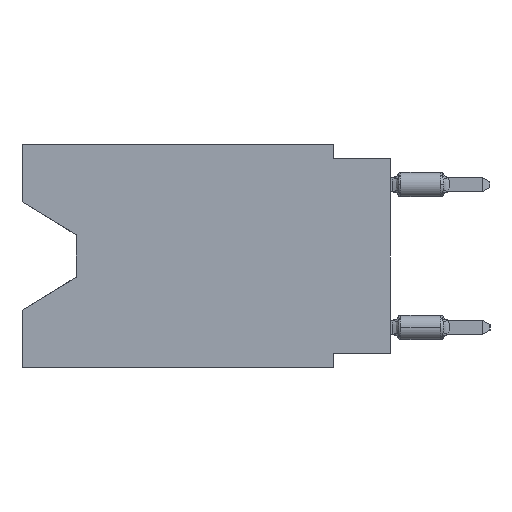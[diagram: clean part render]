
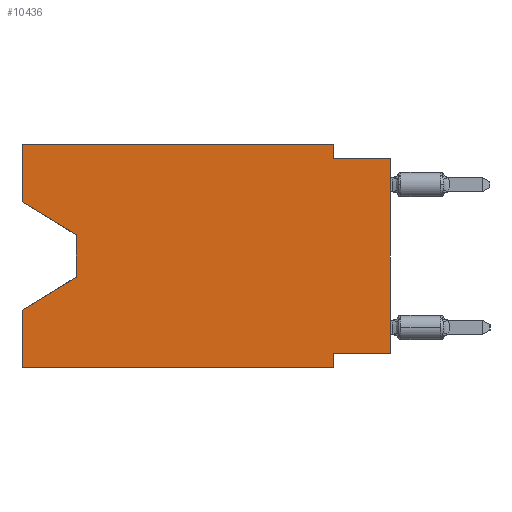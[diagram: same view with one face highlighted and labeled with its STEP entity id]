
A CAD part, left-side view. The second image highlights one B-rep face of the part: STEP entity #10436.
In plain terms, the highlighted planar face has unit normal (-1, 0, 0).
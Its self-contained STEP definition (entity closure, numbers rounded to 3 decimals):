
#299 = VECTOR ( 'NONE', #828, 1000. ) ;
#445 = EDGE_CURVE ( 'NONE', #14486, #13432, #19135, .T. ) ;
#828 = DIRECTION ( 'NONE',  ( 0., 0., -1. ) ) ;
#913 = DIRECTION ( 'NONE',  ( 1., 0., 0. ) ) ;
#1190 = EDGE_CURVE ( 'NONE', #18613, #14375, #9058, .T. ) ;
#1344 = ORIENTED_EDGE ( 'NONE', *, *, #16171, .T. ) ;
#1827 = CARTESIAN_POINT ( 'NONE',  ( 0., 0., 0. ) ) ;
#1930 = DIRECTION ( 'NONE',  ( 0., -1., 0. ) ) ;
#2116 = DIRECTION ( 'NONE',  ( 0., 1., 0. ) ) ;
#2745 = CARTESIAN_POINT ( 'NONE',  ( 0., 16.383, 0. ) ) ;
#3385 = CARTESIAN_POINT ( 'NONE',  ( 0., 2.54, -9.906 ) ) ;
#3682 = CARTESIAN_POINT ( 'NONE',  ( 0., 0., -0.635 ) ) ;
#4029 = PLANE ( 'NONE',  #21563 ) ;
#4590 = LINE ( 'NONE', #11635, #16053 ) ;
#4853 = EDGE_CURVE ( 'NONE', #9731, #14580, #8641, .T. ) ;
#5098 = ORIENTED_EDGE ( 'NONE', *, *, #14408, .F. ) ;
#5248 = CARTESIAN_POINT ( 'NONE',  ( 0., 13.97, -5.893 ) ) ;
#5390 = DIRECTION ( 'NONE',  ( 0., 0., 1. ) ) ;
#5468 = CARTESIAN_POINT ( 'NONE',  ( 0., 16.383, 0. ) ) ;
#5763 = FACE_OUTER_BOUND ( 'NONE', #14326, .T. ) ;
#5974 = DIRECTION ( 'NONE',  ( 0., -0.855, -0.519 ) ) ;
#6468 = VECTOR ( 'NONE', #14177, 1000. ) ;
#6736 = LINE ( 'NONE', #3385, #7605 ) ;
#6860 = VERTEX_POINT ( 'NONE', #8424 ) ;
#7077 = CARTESIAN_POINT ( 'NONE',  ( 0., 16.383, -2.546 ) ) ;
#7278 = ORIENTED_EDGE ( 'NONE', *, *, #10405, .F. ) ;
#7431 = DIRECTION ( 'NONE',  ( 0., 0.855, -0.519 ) ) ;
#7605 = VECTOR ( 'NONE', #15279, 1000. ) ;
#8278 = DIRECTION ( 'NONE',  ( 0., 0., -1. ) ) ;
#8424 = CARTESIAN_POINT ( 'NONE',  ( 0., 13.97, -4.013 ) ) ;
#8461 = ORIENTED_EDGE ( 'NONE', *, *, #18480, .T. ) ;
#8641 = LINE ( 'NONE', #10724, #6468 ) ;
#9058 = LINE ( 'NONE', #5248, #10427 ) ;
#9216 = DIRECTION ( 'NONE',  ( 0., -1., 0. ) ) ;
#9353 = ORIENTED_EDGE ( 'NONE', *, *, #19395, .F. ) ;
#9731 = VERTEX_POINT ( 'NONE', #22059 ) ;
#10322 = ORIENTED_EDGE ( 'NONE', *, *, #21096, .F. ) ;
#10364 = CARTESIAN_POINT ( 'NONE',  ( 0., 16.383, 0. ) ) ;
#10405 = EDGE_CURVE ( 'NONE', #14882, #22396, #19933, .T. ) ;
#10427 = VECTOR ( 'NONE', #7431, 1000. ) ;
#10436 = ADVANCED_FACE ( 'NONE', ( #5763 ), #4029, .F. ) ;
#10542 = EDGE_CURVE ( 'NONE', #14503, #6860, #4590, .T. ) ;
#10724 = CARTESIAN_POINT ( 'NONE',  ( 0., 16.383, -9.906 ) ) ;
#11151 = ORIENTED_EDGE ( 'NONE', *, *, #10542, .T. ) ;
#11308 = EDGE_CURVE ( 'NONE', #13432, #14882, #16746, .T. ) ;
#11338 = CARTESIAN_POINT ( 'NONE',  ( 0., 13.97, -4.013 ) ) ;
#11635 = CARTESIAN_POINT ( 'NONE',  ( 0., 16.383, -2.546 ) ) ;
#11668 = DIRECTION ( 'NONE',  ( 0., 0., -1. ) ) ;
#11767 = CARTESIAN_POINT ( 'NONE',  ( 0., 2.54, 0. ) ) ;
#12210 = CARTESIAN_POINT ( 'NONE',  ( 0., 0., -0.635 ) ) ;
#12446 = CARTESIAN_POINT ( 'NONE',  ( 0., 13.97, -5.893 ) ) ;
#12648 = VECTOR ( 'NONE', #2116, 1000. ) ;
#12834 = VERTEX_POINT ( 'NONE', #13926 ) ;
#12845 = EDGE_CURVE ( 'NONE', #14503, #14486, #15417, .T. ) ;
#13432 = VERTEX_POINT ( 'NONE', #11767 ) ;
#13685 = DIRECTION ( 'NONE',  ( 0., 0., 1. ) ) ;
#13863 = ORIENTED_EDGE ( 'NONE', *, *, #4853, .T. ) ;
#13926 = CARTESIAN_POINT ( 'NONE',  ( 0., 2.54, -9.271 ) ) ;
#14042 = LINE ( 'NONE', #21077, #15215 ) ;
#14177 = DIRECTION ( 'NONE',  ( 0., -1., 0. ) ) ;
#14326 = EDGE_LOOP ( 'NONE', ( #11151, #1344, #22103, #10322, #13863, #5098, #9353, #8461, #7278, #15285, #22270, #18197 ) ) ;
#14375 = VERTEX_POINT ( 'NONE', #20817 ) ;
#14408 = EDGE_CURVE ( 'NONE', #12834, #14580, #6736, .T. ) ;
#14486 = VERTEX_POINT ( 'NONE', #5468 ) ;
#14503 = VERTEX_POINT ( 'NONE', #7077 ) ;
#14580 = VERTEX_POINT ( 'NONE', #21625 ) ;
#14882 = VERTEX_POINT ( 'NONE', #16068 ) ;
#15215 = VECTOR ( 'NONE', #5390, 1000. ) ;
#15279 = DIRECTION ( 'NONE',  ( 0., 0., -1. ) ) ;
#15285 = ORIENTED_EDGE ( 'NONE', *, *, #11308, .F. ) ;
#15286 = CARTESIAN_POINT ( 'NONE',  ( 0., 0., -9.271 ) ) ;
#15417 = LINE ( 'NONE', #22452, #17512 ) ;
#15521 = VERTEX_POINT ( 'NONE', #15286 ) ;
#15835 = CARTESIAN_POINT ( 'NONE',  ( 0., 0., -9.271 ) ) ;
#16053 = VECTOR ( 'NONE', #5974, 1000. ) ;
#16068 = CARTESIAN_POINT ( 'NONE',  ( 0., 2.54, -0.635 ) ) ;
#16171 = EDGE_CURVE ( 'NONE', #6860, #18613, #18371, .T. ) ;
#16746 = LINE ( 'NONE', #22140, #18128 ) ;
#17107 = VECTOR ( 'NONE', #17296, 1000. ) ;
#17296 = DIRECTION ( 'NONE',  ( 0., 0., 1. ) ) ;
#17399 = LINE ( 'NONE', #1827, #17107 ) ;
#17512 = VECTOR ( 'NONE', #13685, 1000. ) ;
#18128 = VECTOR ( 'NONE', #11668, 1000. ) ;
#18197 = ORIENTED_EDGE ( 'NONE', *, *, #12845, .F. ) ;
#18371 = LINE ( 'NONE', #11338, #299 ) ;
#18480 = EDGE_CURVE ( 'NONE', #15521, #22396, #17399, .T. ) ;
#18613 = VERTEX_POINT ( 'NONE', #12446 ) ;
#19135 = LINE ( 'NONE', #10364, #20703 ) ;
#19395 = EDGE_CURVE ( 'NONE', #15521, #12834, #19756, .T. ) ;
#19756 = LINE ( 'NONE', #15835, #12648 ) ;
#19933 = LINE ( 'NONE', #3682, #22653 ) ;
#20703 = VECTOR ( 'NONE', #1930, 1000. ) ;
#20817 = CARTESIAN_POINT ( 'NONE',  ( 0., 16.383, -7.36 ) ) ;
#21077 = CARTESIAN_POINT ( 'NONE',  ( 0., 16.383, 0. ) ) ;
#21096 = EDGE_CURVE ( 'NONE', #9731, #14375, #14042, .T. ) ;
#21563 = AXIS2_PLACEMENT_3D ( 'NONE', #2745, #913, #8278 ) ;
#21625 = CARTESIAN_POINT ( 'NONE',  ( 0., 2.54, -9.906 ) ) ;
#22059 = CARTESIAN_POINT ( 'NONE',  ( 0., 16.383, -9.906 ) ) ;
#22103 = ORIENTED_EDGE ( 'NONE', *, *, #1190, .T. ) ;
#22140 = CARTESIAN_POINT ( 'NONE',  ( 0., 2.54, 0. ) ) ;
#22270 = ORIENTED_EDGE ( 'NONE', *, *, #445, .F. ) ;
#22396 = VERTEX_POINT ( 'NONE', #12210 ) ;
#22452 = CARTESIAN_POINT ( 'NONE',  ( 0., 16.383, 0. ) ) ;
#22653 = VECTOR ( 'NONE', #9216, 1000. ) ;
